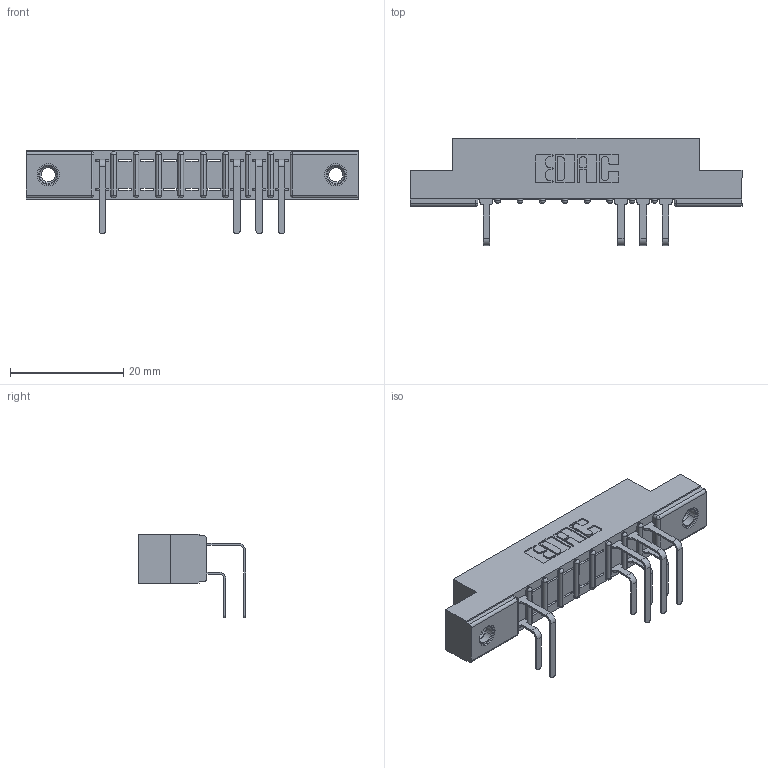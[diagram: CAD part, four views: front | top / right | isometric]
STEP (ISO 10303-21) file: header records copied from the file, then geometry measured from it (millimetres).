
FILE_DESCRIPTION (( 'STEP AP203' ), '1' );
FILE_NAME ('307-009-558-107.STEP', '2018-08-02T20:34:36', ( '' ), ( '' ), 'SwSTEP 2.0', 'SolidWorks 2016', '' );
FILE_SCHEMA (( 'CONFIG_CONTROL_DESIGN' ));
Length unit declared in the file: inch
Products named in the file (5): 307 Part_.156 Dia Mounting Holes; 307-290-001_558 559 - 1 (Single); 307-290-001_558 - 2 (Single); 345-250-001_345-250-005-103; 307-009-558-107
Assembly tree (11 placements, depth 2):
  307-009-558-107
    307 Part_.156 Dia Mounting Holes
    307-290-001_558 559 - 1 (Single)  x4
    307-290-001_558 - 2 (Single)  x4
    345-250-001_345-250-005-103  x2
Bounding box: 58.67 x 18.96 x 14.81 mm (x, y, z)
Volume: 3731.8 mm3; surface area: 5386.6 mm2
Topology: 11 solids, 11 shells, 688 faces, 1915 edges, 1230 vertices
Faces by surface type: plane 426, cylinder 226, sphere 20, cone 12, torus 4
Entity records: 14384 total; most frequent: CARTESIAN_POINT 2392, ORIENTED_EDGE 2370, DIRECTION 2355, EDGE_CURVE 1185, LINE 893, VECTOR 893, VERTEX_POINT 768, AXIS2_PLACEMENT_3D 731
